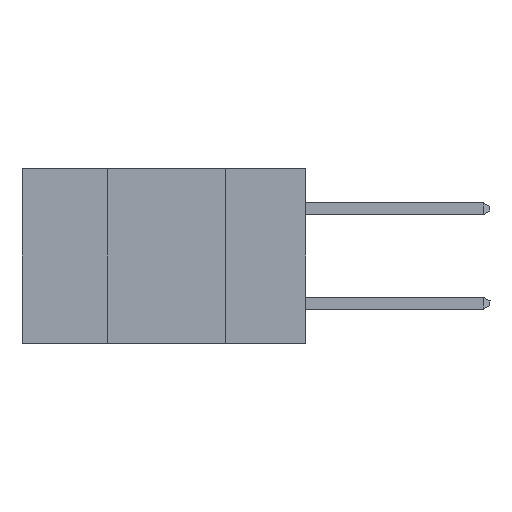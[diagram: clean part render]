
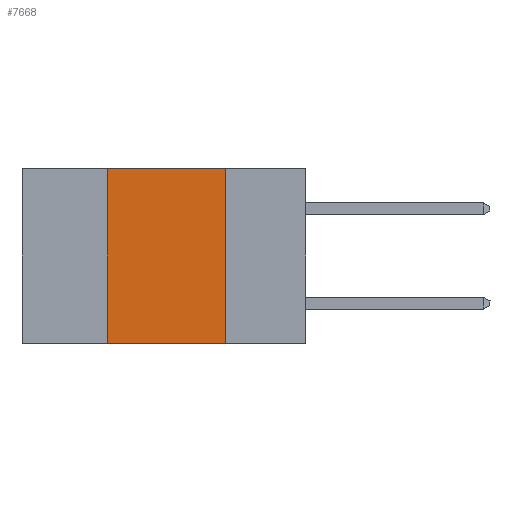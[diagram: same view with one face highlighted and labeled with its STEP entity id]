
A CAD part, left-side view. The second image highlights one B-rep face of the part: STEP entity #7668.
In plain terms, the highlighted planar face has unit normal (-1, 0, 0).
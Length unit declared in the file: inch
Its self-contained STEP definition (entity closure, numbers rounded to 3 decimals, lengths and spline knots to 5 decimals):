
#185 = VERTEX_POINT ( 'NONE', #9984 ) ;
#1707 = EDGE_CURVE ( 'NONE', #2483, #2842, #8010, .T. ) ;
#2316 = EDGE_CURVE ( 'NONE', #185, #8306, #4123, .T. ) ;
#2483 = VERTEX_POINT ( 'NONE', #4608 ) ;
#2489 = ORIENTED_EDGE ( 'NONE', *, *, #5831, .F. ) ;
#2659 = VECTOR ( 'NONE', #7758, 39.37008 ) ;
#2842 = VERTEX_POINT ( 'NONE', #5734 ) ;
#3225 = PLANE ( 'NONE',  #9314 ) ;
#3238 = CARTESIAN_POINT ( 'NONE',  ( 0., 0.17, -0.37 ) ) ;
#3969 = FACE_OUTER_BOUND ( 'NONE', #4396, .T. ) ;
#4010 = DIRECTION ( 'NONE',  ( 0., 0., -1. ) ) ;
#4123 = LINE ( 'NONE', #9585, #5976 ) ;
#4396 = EDGE_LOOP ( 'NONE', ( #2489, #5973, #6958, #8548 ) ) ;
#4495 = VECTOR ( 'NONE', #5289, 39.37008 ) ;
#4572 = CARTESIAN_POINT ( 'NONE',  ( 0., 0.42, 0. ) ) ;
#4608 = CARTESIAN_POINT ( 'NONE',  ( 0., 0.42, 0. ) ) ;
#5074 = CARTESIAN_POINT ( 'NONE',  ( 0., 0.17, 0. ) ) ;
#5289 = DIRECTION ( 'NONE',  ( 0., 0., -1. ) ) ;
#5734 = CARTESIAN_POINT ( 'NONE',  ( 0., 0.17, 0. ) ) ;
#5831 = EDGE_CURVE ( 'NONE', #2842, #8306, #7158, .T. ) ;
#5973 = ORIENTED_EDGE ( 'NONE', *, *, #1707, .F. ) ;
#5976 = VECTOR ( 'NONE', #7938, 39.37008 ) ;
#6189 = DIRECTION ( 'NONE',  ( 0., 0., 1. ) ) ;
#6958 = ORIENTED_EDGE ( 'NONE', *, *, #9129, .F. ) ;
#7158 = LINE ( 'NONE', #5074, #4495 ) ;
#7668 = ADVANCED_FACE ( 'NONE', ( #3969 ), #3225, .F. ) ;
#7758 = DIRECTION ( 'NONE',  ( 0., -1., 0. ) ) ;
#7938 = DIRECTION ( 'NONE',  ( 0., -1., 0. ) ) ;
#8010 = LINE ( 'NONE', #10087, #2659 ) ;
#8066 = VECTOR ( 'NONE', #6189, 39.37008 ) ;
#8306 = VERTEX_POINT ( 'NONE', #3238 ) ;
#8548 = ORIENTED_EDGE ( 'NONE', *, *, #2316, .T. ) ;
#8658 = DIRECTION ( 'NONE',  ( 1., 0., 0. ) ) ;
#9129 = EDGE_CURVE ( 'NONE', #185, #2483, #9929, .T. ) ;
#9314 = AXIS2_PLACEMENT_3D ( 'NONE', #9505, #8658, #4010 ) ;
#9505 = CARTESIAN_POINT ( 'NONE',  ( 0., 0.6, 0. ) ) ;
#9585 = CARTESIAN_POINT ( 'NONE',  ( 0., 0.6, -0.37 ) ) ;
#9929 = LINE ( 'NONE', #4572, #8066 ) ;
#9984 = CARTESIAN_POINT ( 'NONE',  ( 0., 0.42, -0.37 ) ) ;
#10087 = CARTESIAN_POINT ( 'NONE',  ( 0., 0.6, 0. ) ) ;
